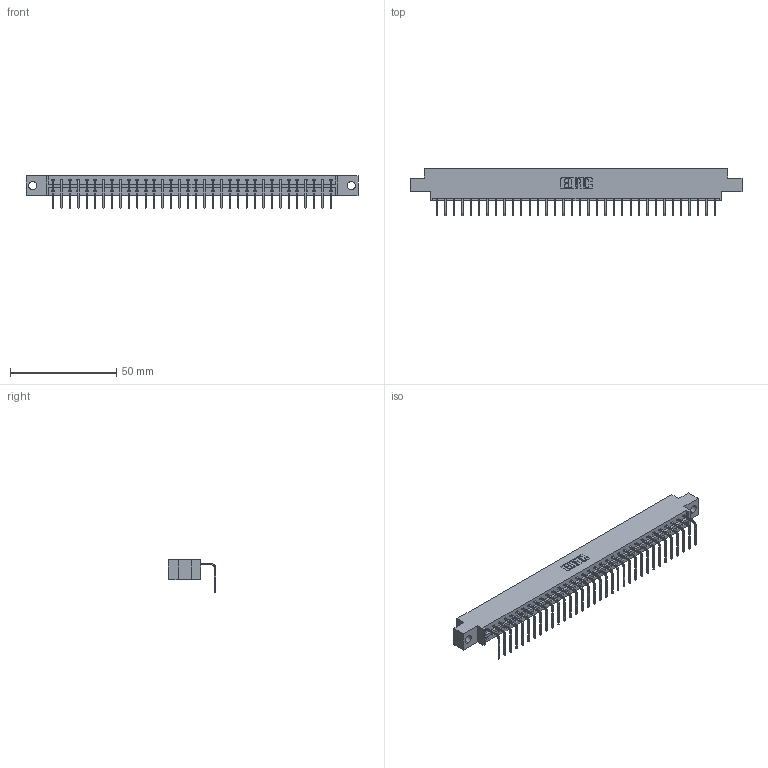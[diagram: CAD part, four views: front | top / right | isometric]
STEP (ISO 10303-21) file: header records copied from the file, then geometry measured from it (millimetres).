
FILE_DESCRIPTION (( 'STEP AP203' ), '1' );
FILE_NAME ('333-034-558-604.STEP', '2018-08-02T22:57:58', ( '' ), ( '' ), 'SwSTEP 2.0', 'SolidWorks 2016', '' );
FILE_SCHEMA (( 'CONFIG_CONTROL_DESIGN' ));
Length unit declared in the file: inch
Products named in the file (3): 333 Part_Offset - .156 Dia - TH; 345-292-001_558 Tail - 2; 333-034-558-604
Assembly tree (35 placements, depth 2):
  333-034-558-604
    333 Part_Offset - .156 Dia - TH
    345-292-001_558 Tail - 2  x34
Bounding box: 156.26 x 22.17 x 15.37 mm (x, y, z)
Volume: 15453.1 mm3; surface area: 17355.6 mm2
Topology: 35 solids, 35 shells, 2158 faces, 6511 edges, 4294 vertices
Faces by surface type: plane 1570, cylinder 588
Entity records: 22039 total; most frequent: CARTESIAN_POINT 3812, ORIENTED_EDGE 3782, DIRECTION 3231, EDGE_CURVE 1891, LINE 1763, VECTOR 1763, VERTEX_POINT 1258, AXIS2_PLACEMENT_3D 734
